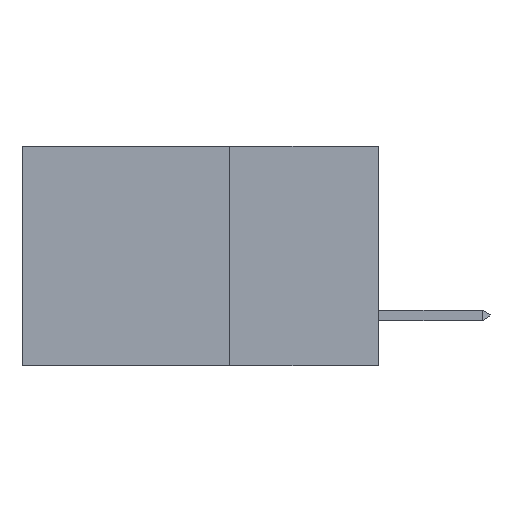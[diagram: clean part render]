
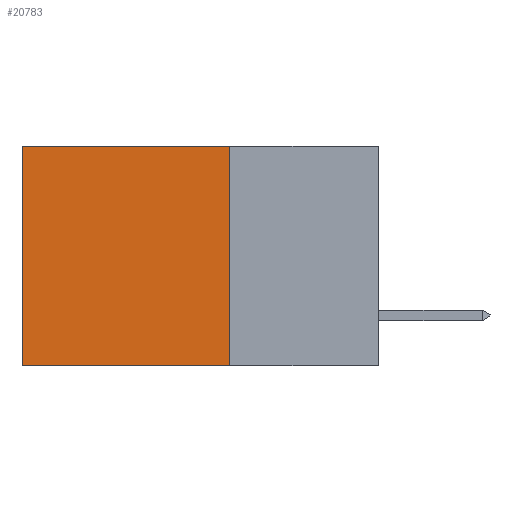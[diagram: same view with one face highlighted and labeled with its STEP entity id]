
A CAD part, left-side view. The second image highlights one B-rep face of the part: STEP entity #20783.
In plain terms, the highlighted planar face has unit normal (-1, 0, 0).
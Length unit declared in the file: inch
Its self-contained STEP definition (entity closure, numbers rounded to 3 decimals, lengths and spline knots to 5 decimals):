
#333 = ORIENTED_EDGE ( 'NONE', *, *, #8627, .T. ) ;
#873 = EDGE_CURVE ( 'NONE', #16680, #13074, #17419, .T. ) ;
#1434 = LINE ( 'NONE', #12167, #18089 ) ;
#1997 = CARTESIAN_POINT ( 'NONE',  ( 0.298, 0.25, 0. ) ) ;
#2071 = VECTOR ( 'NONE', #11283, 39.37008 ) ;
#2959 = VECTOR ( 'NONE', #12233, 39.37008 ) ;
#4565 = LINE ( 'NONE', #9816, #16938 ) ;
#6068 = AXIS2_PLACEMENT_3D ( 'NONE', #1997, #19672, #17844 ) ;
#6702 = PLANE ( 'NONE',  #6068 ) ;
#8542 = EDGE_CURVE ( 'NONE', #13074, #20341, #12089, .T. ) ;
#8627 = EDGE_CURVE ( 'NONE', #20624, #20341, #1434, .T. ) ;
#9339 = ORIENTED_EDGE ( 'NONE', *, *, #8542, .F. ) ;
#9816 = CARTESIAN_POINT ( 'NONE',  ( 0.298, 0.25, 0. ) ) ;
#10449 = DIRECTION ( 'NONE',  ( 0., 0., -1. ) ) ;
#10635 = CARTESIAN_POINT ( 'NONE',  ( 0.298, 0.6, 0. ) ) ;
#11283 = DIRECTION ( 'NONE',  ( 0., 0., -1. ) ) ;
#12089 = LINE ( 'NONE', #18478, #2959 ) ;
#12167 = CARTESIAN_POINT ( 'NONE',  ( 0.298, 0.6, 0. ) ) ;
#12233 = DIRECTION ( 'NONE',  ( 0., 1., 0. ) ) ;
#12916 = CARTESIAN_POINT ( 'NONE',  ( 0.298, 0.6, -0.37 ) ) ;
#13074 = VERTEX_POINT ( 'NONE', #16619 ) ;
#13774 = FACE_OUTER_BOUND ( 'NONE', #17380, .T. ) ;
#15059 = EDGE_CURVE ( 'NONE', #16680, #20624, #4565, .T. ) ;
#16619 = CARTESIAN_POINT ( 'NONE',  ( 0.298, 0.25, -0.37 ) ) ;
#16680 = VERTEX_POINT ( 'NONE', #20498 ) ;
#16938 = VECTOR ( 'NONE', #19289, 39.37008 ) ;
#17380 = EDGE_LOOP ( 'NONE', ( #333, #9339, #19766, #18667 ) ) ;
#17419 = LINE ( 'NONE', #17664, #2071 ) ;
#17664 = CARTESIAN_POINT ( 'NONE',  ( 0.298, 0.25, 0. ) ) ;
#17844 = DIRECTION ( 'NONE',  ( 0., 0., -1. ) ) ;
#18089 = VECTOR ( 'NONE', #10449, 39.37008 ) ;
#18478 = CARTESIAN_POINT ( 'NONE',  ( 0.298, 0.25, -0.37 ) ) ;
#18667 = ORIENTED_EDGE ( 'NONE', *, *, #15059, .T. ) ;
#19289 = DIRECTION ( 'NONE',  ( 0., 1., 0. ) ) ;
#19672 = DIRECTION ( 'NONE',  ( 1., 0., 0. ) ) ;
#19766 = ORIENTED_EDGE ( 'NONE', *, *, #873, .F. ) ;
#20341 = VERTEX_POINT ( 'NONE', #12916 ) ;
#20498 = CARTESIAN_POINT ( 'NONE',  ( 0.298, 0.25, 0. ) ) ;
#20624 = VERTEX_POINT ( 'NONE', #10635 ) ;
#20783 = ADVANCED_FACE ( 'NONE', ( #13774 ), #6702, .F. ) ;
